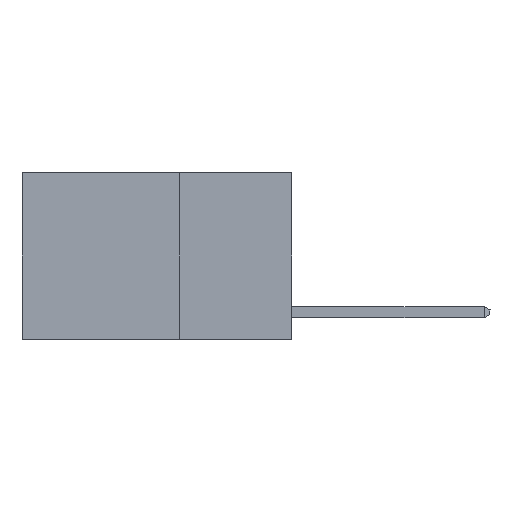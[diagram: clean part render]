
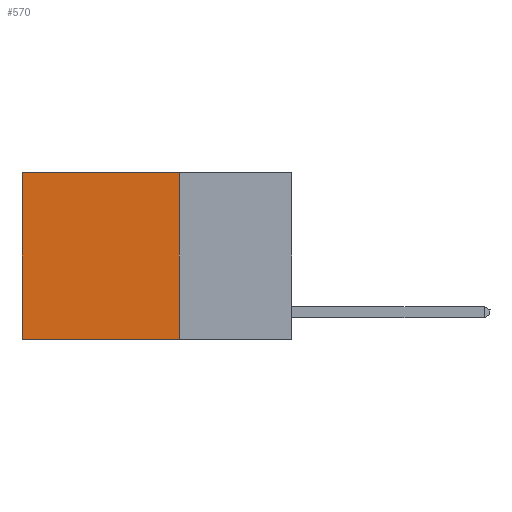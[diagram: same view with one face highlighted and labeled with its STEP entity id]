
A CAD part, left-side view. The second image highlights one B-rep face of the part: STEP entity #570.
In plain terms, the highlighted planar face has unit normal (-1, 0, 0).
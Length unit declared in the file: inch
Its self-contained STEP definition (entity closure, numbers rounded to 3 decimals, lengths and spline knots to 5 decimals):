
#206 = LINE ( 'NONE', #15997, #13797 ) ;
#570 = ADVANCED_FACE ( 'NONE', ( #14295 ), #5251, .F. ) ;
#645 = DIRECTION ( 'NONE',  ( 0., 1., 0. ) ) ;
#1079 = CARTESIAN_POINT ( 'NONE',  ( 0.2625, 0.25, 0. ) ) ;
#1485 = EDGE_CURVE ( 'NONE', #14495, #13157, #7382, .T. ) ;
#1607 = CARTESIAN_POINT ( 'NONE',  ( 0.2625, 0.6, 0. ) ) ;
#2017 = VECTOR ( 'NONE', #645, 39.37008 ) ;
#2098 = LINE ( 'NONE', #2629, #16027 ) ;
#2437 = CARTESIAN_POINT ( 'NONE',  ( 0.2625, 0.6, -0.37 ) ) ;
#2442 = LINE ( 'NONE', #14207, #2017 ) ;
#2629 = CARTESIAN_POINT ( 'NONE',  ( 0.2625, 0.25, 0. ) ) ;
#3779 = VECTOR ( 'NONE', #12427, 39.37008 ) ;
#4012 = DIRECTION ( 'NONE',  ( 0., 1., 0. ) ) ;
#5251 = PLANE ( 'NONE',  #5651 ) ;
#5312 = VERTEX_POINT ( 'NONE', #5933 ) ;
#5651 = AXIS2_PLACEMENT_3D ( 'NONE', #1079, #16003, #7956 ) ;
#5933 = CARTESIAN_POINT ( 'NONE',  ( 0.2625, 0.25, 0. ) ) ;
#6595 = DIRECTION ( 'NONE',  ( 0., 0., -1. ) ) ;
#6960 = EDGE_LOOP ( 'NONE', ( #13410, #16347, #15087, #15981 ) ) ;
#7382 = LINE ( 'NONE', #1607, #3779 ) ;
#7956 = DIRECTION ( 'NONE',  ( 0., 0., -1. ) ) ;
#10060 = CARTESIAN_POINT ( 'NONE',  ( 0.2625, 0.25, -0.37 ) ) ;
#12427 = DIRECTION ( 'NONE',  ( 0., 0., -1. ) ) ;
#12686 = EDGE_CURVE ( 'NONE', #5312, #14495, #2098, .T. ) ;
#13157 = VERTEX_POINT ( 'NONE', #2437 ) ;
#13410 = ORIENTED_EDGE ( 'NONE', *, *, #1485, .T. ) ;
#13797 = VECTOR ( 'NONE', #6595, 39.37008 ) ;
#14207 = CARTESIAN_POINT ( 'NONE',  ( 0.2625, 0.25, -0.37 ) ) ;
#14295 = FACE_OUTER_BOUND ( 'NONE', #6960, .T. ) ;
#14495 = VERTEX_POINT ( 'NONE', #16004 ) ;
#14833 = VERTEX_POINT ( 'NONE', #10060 ) ;
#14936 = EDGE_CURVE ( 'NONE', #14833, #13157, #2442, .T. ) ;
#15087 = ORIENTED_EDGE ( 'NONE', *, *, #16462, .F. ) ;
#15981 = ORIENTED_EDGE ( 'NONE', *, *, #12686, .T. ) ;
#15997 = CARTESIAN_POINT ( 'NONE',  ( 0.2625, 0.25, 0. ) ) ;
#16003 = DIRECTION ( 'NONE',  ( 1., 0., 0. ) ) ;
#16004 = CARTESIAN_POINT ( 'NONE',  ( 0.2625, 0.6, 0. ) ) ;
#16027 = VECTOR ( 'NONE', #4012, 39.37008 ) ;
#16347 = ORIENTED_EDGE ( 'NONE', *, *, #14936, .F. ) ;
#16462 = EDGE_CURVE ( 'NONE', #5312, #14833, #206, .T. ) ;
